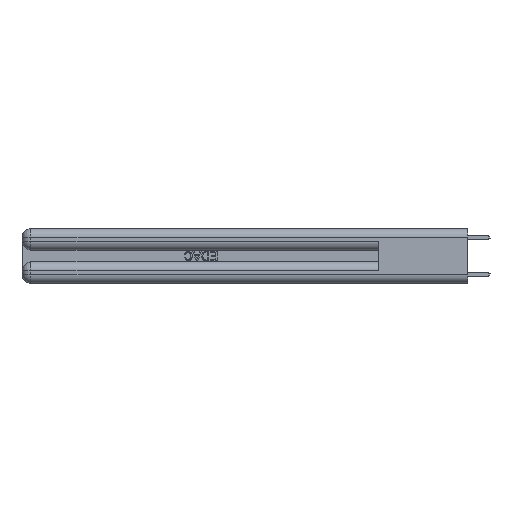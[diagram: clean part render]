
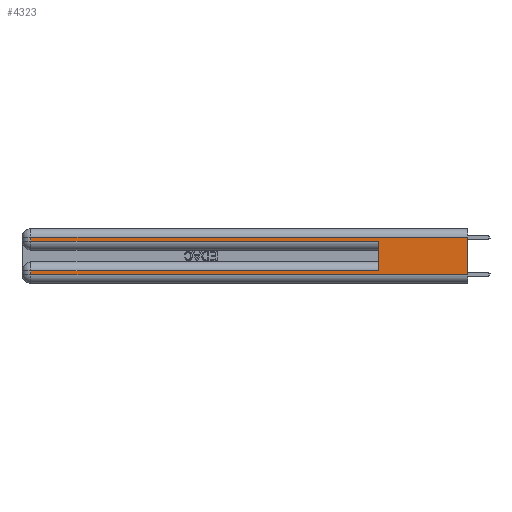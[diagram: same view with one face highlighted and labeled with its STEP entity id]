
A CAD part, left-side view. The second image highlights one B-rep face of the part: STEP entity #4323.
In plain terms, the highlighted planar face has unit normal (-1, 0, 0).
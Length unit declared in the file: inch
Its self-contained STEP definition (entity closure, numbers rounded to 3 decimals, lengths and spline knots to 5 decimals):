
#1801 = VERTEX_POINT ( 'NONE', #20433 ) ;
#2736 = LINE ( 'NONE', #27245, #4585 ) ;
#3824 = VECTOR ( 'NONE', #19384, 39.37008 ) ;
#3968 = ORIENTED_EDGE ( 'NONE', *, *, #30120, .T. ) ;
#4152 = ORIENTED_EDGE ( 'NONE', *, *, #7451, .T. ) ;
#4323 = ADVANCED_FACE ( 'NONE', ( #21813 ), #13377, .F. ) ;
#4381 = CARTESIAN_POINT ( 'NONE',  ( 0., 2.94, 0.085 ) ) ;
#4401 = VERTEX_POINT ( 'NONE', #14972 ) ;
#4585 = VECTOR ( 'NONE', #8167, 39.37008 ) ;
#4886 = ORIENTED_EDGE ( 'NONE', *, *, #18991, .T. ) ;
#5628 = CARTESIAN_POINT ( 'NONE',  ( 0., 0.6, 0.145 ) ) ;
#5880 = EDGE_CURVE ( 'NONE', #23455, #35505, #19244, .T. ) ;
#6469 = LINE ( 'NONE', #17090, #14924 ) ;
#6799 = EDGE_CURVE ( 'NONE', #30712, #1801, #13556, .T. ) ;
#7451 = EDGE_CURVE ( 'NONE', #15081, #1801, #8999, .T. ) ;
#8167 = DIRECTION ( 'NONE',  ( 0., -1., 0. ) ) ;
#8417 = CARTESIAN_POINT ( 'NONE',  ( 0., 0., 0.31 ) ) ;
#8441 = VECTOR ( 'NONE', #17096, 39.37008 ) ;
#8999 = LINE ( 'NONE', #22846, #8441 ) ;
#10448 = CARTESIAN_POINT ( 'NONE',  ( 0., 2.94, 0.31 ) ) ;
#10733 = DIRECTION ( 'NONE',  ( 0., 0., -1. ) ) ;
#11997 = CARTESIAN_POINT ( 'NONE',  ( 0., 0., 0.06 ) ) ;
#12395 = VECTOR ( 'NONE', #10733, 39.37008 ) ;
#12427 = VECTOR ( 'NONE', #26795, 39.37008 ) ;
#12585 = VECTOR ( 'NONE', #18904, 39.37008 ) ;
#13040 = CARTESIAN_POINT ( 'NONE',  ( 0., 0.6, 0.085 ) ) ;
#13377 = PLANE ( 'NONE',  #16180 ) ;
#13556 = LINE ( 'NONE', #5628, #21473 ) ;
#14370 = LINE ( 'NONE', #8417, #3824 ) ;
#14924 = VECTOR ( 'NONE', #30812, 39.37008 ) ;
#14972 = CARTESIAN_POINT ( 'NONE',  ( 0., 0., 0.31 ) ) ;
#15081 = VERTEX_POINT ( 'NONE', #33119 ) ;
#16180 = AXIS2_PLACEMENT_3D ( 'NONE', #24327, #21635, #18940 ) ;
#17090 = CARTESIAN_POINT ( 'NONE',  ( 0., 2.94, 0.37 ) ) ;
#17096 = DIRECTION ( 'NONE',  ( 0., -1., 0. ) ) ;
#17789 = ORIENTED_EDGE ( 'NONE', *, *, #5880, .T. ) ;
#18227 = EDGE_CURVE ( 'NONE', #34609, #15081, #6469, .T. ) ;
#18904 = DIRECTION ( 'NONE',  ( 0., 0., -1. ) ) ;
#18940 = DIRECTION ( 'NONE',  ( 0., 0., -1. ) ) ;
#18991 = EDGE_CURVE ( 'NONE', #35505, #20419, #2736, .T. ) ;
#19244 = LINE ( 'NONE', #33367, #12585 ) ;
#19384 = DIRECTION ( 'NONE',  ( 0., 1., 0. ) ) ;
#19752 = EDGE_LOOP ( 'NONE', ( #27385, #3968, #33226, #4152, #30095, #30124, #17789, #4886 ) ) ;
#20419 = VERTEX_POINT ( 'NONE', #11997 ) ;
#20433 = CARTESIAN_POINT ( 'NONE',  ( 0., 0.6, 0.285 ) ) ;
#21473 = VECTOR ( 'NONE', #22354, 39.37008 ) ;
#21635 = DIRECTION ( 'NONE',  ( 1., 0., 0. ) ) ;
#21813 = FACE_OUTER_BOUND ( 'NONE', #19752, .T. ) ;
#22354 = DIRECTION ( 'NONE',  ( 0., 0., 1. ) ) ;
#22846 = CARTESIAN_POINT ( 'NONE',  ( 0., 0., 0.285 ) ) ;
#23039 = CARTESIAN_POINT ( 'NONE',  ( 0., 2.94, 0.06 ) ) ;
#23455 = VERTEX_POINT ( 'NONE', #4381 ) ;
#24327 = CARTESIAN_POINT ( 'NONE',  ( 0., 0., 0.37 ) ) ;
#24421 = LINE ( 'NONE', #34965, #12427 ) ;
#26795 = DIRECTION ( 'NONE',  ( 0., 1., 0. ) ) ;
#27245 = CARTESIAN_POINT ( 'NONE',  ( 0., 0., 0.06 ) ) ;
#27385 = ORIENTED_EDGE ( 'NONE', *, *, #29265, .F. ) ;
#27824 = LINE ( 'NONE', #35451, #12395 ) ;
#29265 = EDGE_CURVE ( 'NONE', #4401, #20419, #27824, .T. ) ;
#30003 = EDGE_CURVE ( 'NONE', #30712, #23455, #24421, .T. ) ;
#30095 = ORIENTED_EDGE ( 'NONE', *, *, #6799, .F. ) ;
#30120 = EDGE_CURVE ( 'NONE', #4401, #34609, #14370, .T. ) ;
#30124 = ORIENTED_EDGE ( 'NONE', *, *, #30003, .T. ) ;
#30712 = VERTEX_POINT ( 'NONE', #13040 ) ;
#30812 = DIRECTION ( 'NONE',  ( 0., 0., -1. ) ) ;
#33119 = CARTESIAN_POINT ( 'NONE',  ( 0., 2.94, 0.285 ) ) ;
#33226 = ORIENTED_EDGE ( 'NONE', *, *, #18227, .T. ) ;
#33367 = CARTESIAN_POINT ( 'NONE',  ( 0., 2.94, 0.37 ) ) ;
#34609 = VERTEX_POINT ( 'NONE', #10448 ) ;
#34965 = CARTESIAN_POINT ( 'NONE',  ( 0., 0., 0.085 ) ) ;
#35451 = CARTESIAN_POINT ( 'NONE',  ( 0., 0., 0.37 ) ) ;
#35505 = VERTEX_POINT ( 'NONE', #23039 ) ;
